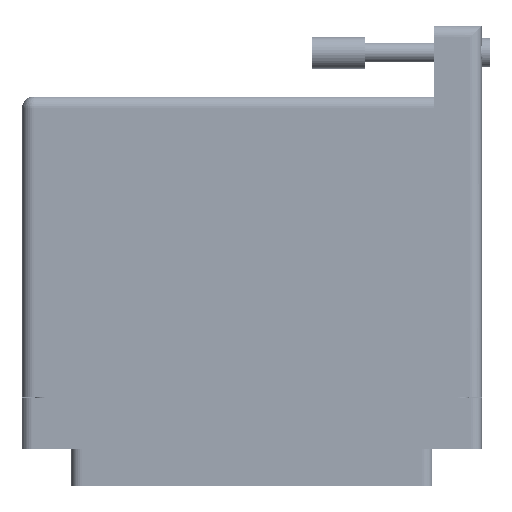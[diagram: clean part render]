
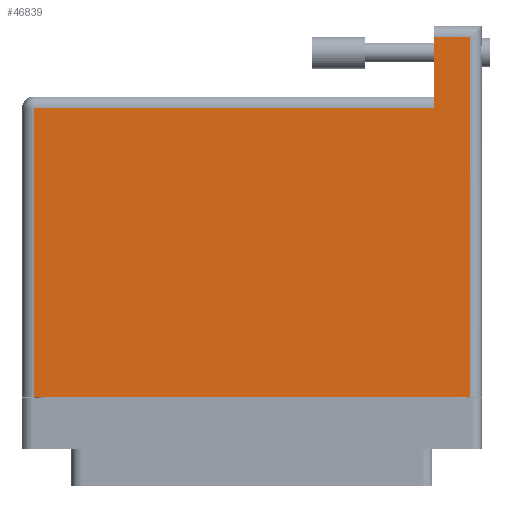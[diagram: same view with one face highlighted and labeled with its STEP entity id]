
A CAD part, front view. The second image highlights one B-rep face of the part: STEP entity #46839.
In plain terms, the highlighted face is planar.
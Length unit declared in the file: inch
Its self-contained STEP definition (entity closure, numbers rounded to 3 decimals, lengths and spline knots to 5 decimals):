
#215 = CARTESIAN_POINT ( 'NONE',  ( -1.359, 2.025, 0.617 ) ) ;
#1398 = DIRECTION ( 'NONE',  ( -1., 0., 0. ) ) ;
#1546 = ORIENTED_EDGE ( 'NONE', *, *, #36992, .T. ) ;
#4317 = VERTEX_POINT ( 'NONE', #25339 ) ;
#5459 = CARTESIAN_POINT ( 'NONE',  ( 1.289, -0.1, 0.617 ) ) ;
#6413 = LINE ( 'NONE', #69543, #66933 ) ;
#7772 = ORIENTED_EDGE ( 'NONE', *, *, #39720, .T. ) ;
#8299 = CARTESIAN_POINT ( 'NONE',  ( 1.079, 2.025, 0.617 ) ) ;
#9383 = VERTEX_POINT ( 'NONE', #8299 ) ;
#11390 = VERTEX_POINT ( 'NONE', #40969 ) ;
#13461 = DIRECTION ( 'NONE',  ( 1., 0., 0. ) ) ;
#19188 = ORIENTED_EDGE ( 'NONE', *, *, #32059, .T. ) ;
#20320 = CARTESIAN_POINT ( 'NONE',  ( 1.289, 2.095, 0.617 ) ) ;
#21059 = EDGE_CURVE ( 'NONE', #9383, #4317, #41358, .T. ) ;
#22819 = VECTOR ( 'NONE', #13461, 39.37008 ) ;
#23925 = CARTESIAN_POINT ( 'NONE',  ( 1.289, 2.025, 0.617 ) ) ;
#25339 = CARTESIAN_POINT ( 'NONE',  ( 1.079, 1.605, 0.617 ) ) ;
#25452 = VECTOR ( 'NONE', #61908, 39.37008 ) ;
#26427 = LINE ( 'NONE', #62987, #22819 ) ;
#28714 = CARTESIAN_POINT ( 'NONE',  ( -1.289, -0.1, 0.617 ) ) ;
#30058 = VERTEX_POINT ( 'NONE', #28714 ) ;
#31485 = DIRECTION ( 'NONE',  ( -1., 0., 0. ) ) ;
#32059 = EDGE_CURVE ( 'NONE', #40230, #9383, #63745, .T. ) ;
#32395 = VECTOR ( 'NONE', #71606, 39.37008 ) ;
#35169 = ORIENTED_EDGE ( 'NONE', *, *, #60368, .T. ) ;
#36992 = EDGE_CURVE ( 'NONE', #30058, #44543, #26427, .T. ) ;
#39720 = EDGE_CURVE ( 'NONE', #4317, #11390, #54458, .T. ) ;
#40230 = VERTEX_POINT ( 'NONE', #23925 ) ;
#40969 = CARTESIAN_POINT ( 'NONE',  ( -1.289, 1.605, 0.617 ) ) ;
#40973 = DIRECTION ( 'NONE',  ( 0., 0., -1. ) ) ;
#41358 = LINE ( 'NONE', #43573, #32395 ) ;
#41628 = LINE ( 'NONE', #20320, #65596 ) ;
#42011 = AXIS2_PLACEMENT_3D ( 'NONE', #48544, #40973, #1398 ) ;
#43573 = CARTESIAN_POINT ( 'NONE',  ( 1.079, 2.095, 0.617 ) ) ;
#43830 = FACE_OUTER_BOUND ( 'NONE', #59801, .T. ) ;
#44543 = VERTEX_POINT ( 'NONE', #5459 ) ;
#45275 = PLANE ( 'NONE',  #42011 ) ;
#46239 = EDGE_CURVE ( 'NONE', #11390, #30058, #6413, .T. ) ;
#46839 = ADVANCED_FACE ( 'NONE', ( #43830 ), #45275, .F. ) ;
#48351 = ORIENTED_EDGE ( 'NONE', *, *, #21059, .T. ) ;
#48544 = CARTESIAN_POINT ( 'NONE',  ( -1.359, 1.675, 0.617 ) ) ;
#48570 = ORIENTED_EDGE ( 'NONE', *, *, #46239, .T. ) ;
#53203 = DIRECTION ( 'NONE',  ( 0., -1., 0. ) ) ;
#54458 = LINE ( 'NONE', #54971, #57964 ) ;
#54971 = CARTESIAN_POINT ( 'NONE',  ( -1.359, 1.605, 0.617 ) ) ;
#54972 = DIRECTION ( 'NONE',  ( 0., 1., 0. ) ) ;
#57964 = VECTOR ( 'NONE', #31485, 39.37008 ) ;
#59801 = EDGE_LOOP ( 'NONE', ( #7772, #48570, #1546, #35169, #19188, #48351 ) ) ;
#60368 = EDGE_CURVE ( 'NONE', #44543, #40230, #41628, .T. ) ;
#61908 = DIRECTION ( 'NONE',  ( -1., 0., 0. ) ) ;
#62987 = CARTESIAN_POINT ( 'NONE',  ( -1.359, -0.1, 0.617 ) ) ;
#63745 = LINE ( 'NONE', #215, #25452 ) ;
#65596 = VECTOR ( 'NONE', #54972, 39.37008 ) ;
#66933 = VECTOR ( 'NONE', #53203, 39.37008 ) ;
#69543 = CARTESIAN_POINT ( 'NONE',  ( -1.289, -0.1, 0.617 ) ) ;
#71606 = DIRECTION ( 'NONE',  ( 0., -1., 0. ) ) ;
